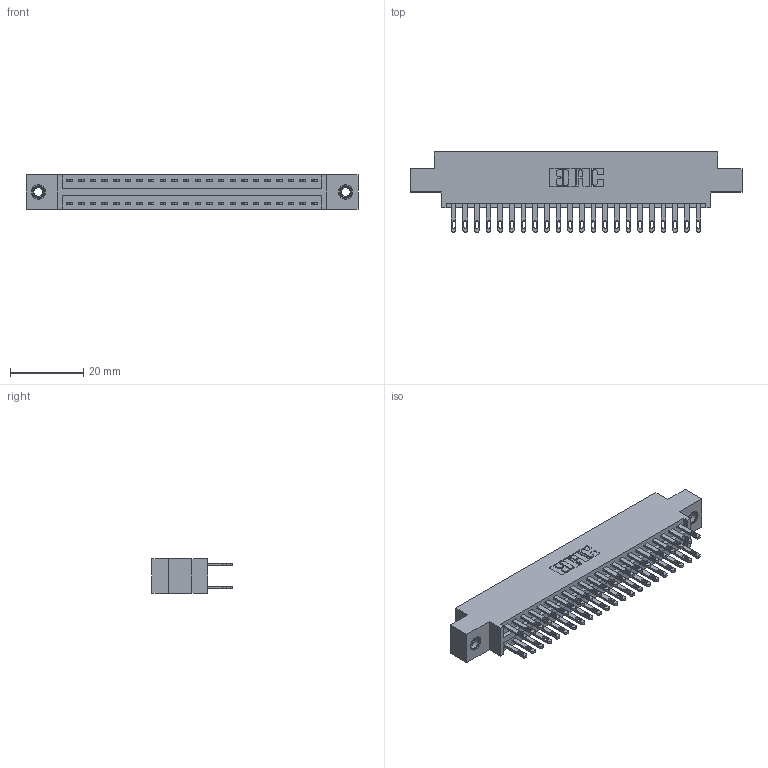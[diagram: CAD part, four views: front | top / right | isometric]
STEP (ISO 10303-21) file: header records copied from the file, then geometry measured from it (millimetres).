
FILE_DESCRIPTION (( 'STEP AP203' ), '1' );
FILE_NAME ('346-044-500-807.STEP', '2018-08-25T00:53:18', ( '' ), ( '' ), 'SwSTEP 2.0', 'SolidWorks 2016', '' );
FILE_SCHEMA (( 'CONFIG_CONTROL_DESIGN' ));
Length unit declared in the file: inch
Products named in the file (4): 346-044-500-807; 346 Part_0.170 Offset - 0.156 Dia-TI; 345-292-001_345-293-100; 345-250-001_345-250-005-103
Assembly tree (47 placements, depth 2):
  346-044-500-807
    346 Part_0.170 Offset - 0.156 Dia-TI
    345-292-001_345-293-100  x44
    345-250-001_345-250-005-103  x2
Bounding box: 90.42 x 21.84 x 9.4 mm (x, y, z)
Volume: 8628.5 mm3; surface area: 12219.9 mm2
Topology: 47 solids, 47 shells, 2298 faces, 6945 edges, 4622 vertices
Faces by surface type: plane 1388, cylinder 894, cone 12, torus 4
Entity records: 18298 total; most frequent: CARTESIAN_POINT 3027, ORIENTED_EDGE 2954, DIRECTION 2747, EDGE_CURVE 1477, VECTOR 1233, LINE 1233, VERTEX_POINT 980, AXIS2_PLACEMENT_3D 757
